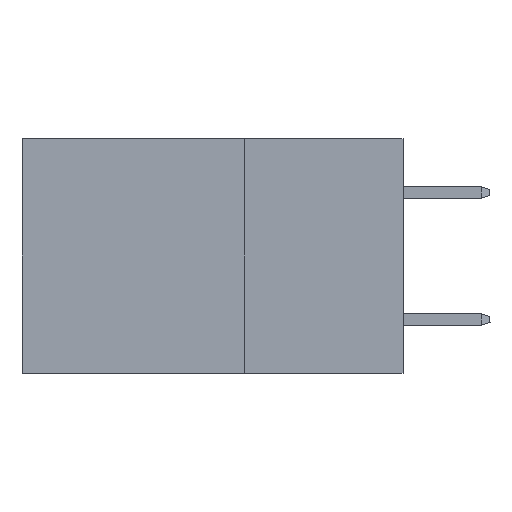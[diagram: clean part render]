
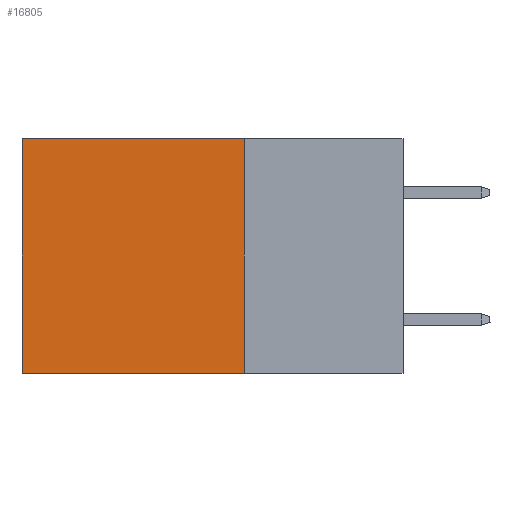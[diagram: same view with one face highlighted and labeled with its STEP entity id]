
A CAD part, left-side view. The second image highlights one B-rep face of the part: STEP entity #16805.
In plain terms, the highlighted planar face has unit normal (-1, 0, 0).
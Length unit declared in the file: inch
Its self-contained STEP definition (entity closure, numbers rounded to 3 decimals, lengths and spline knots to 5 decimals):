
#731 = CARTESIAN_POINT ( 'NONE',  ( 0.2875, 0.25, -0.37 ) ) ;
#1231 = EDGE_CURVE ( 'NONE', #6450, #15785, #3109, .T. ) ;
#1789 = VECTOR ( 'NONE', #8354, 39.37008 ) ;
#1845 = DIRECTION ( 'NONE',  ( 0., 0., -1. ) ) ;
#2257 = CARTESIAN_POINT ( 'NONE',  ( 0.2875, 0.25, -0.37 ) ) ;
#2353 = LINE ( 'NONE', #10045, #1789 ) ;
#3051 = AXIS2_PLACEMENT_3D ( 'NONE', #13558, #13741, #1845 ) ;
#3069 = CARTESIAN_POINT ( 'NONE',  ( 0.2875, 0.6, 0. ) ) ;
#3109 = LINE ( 'NONE', #10684, #17189 ) ;
#4097 = EDGE_CURVE ( 'NONE', #10694, #15785, #6699, .T. ) ;
#6450 = VERTEX_POINT ( 'NONE', #3069 ) ;
#6531 = ORIENTED_EDGE ( 'NONE', *, *, #14294, .F. ) ;
#6699 = LINE ( 'NONE', #2257, #8465 ) ;
#6700 = CARTESIAN_POINT ( 'NONE',  ( 0.2875, 0.25, 0. ) ) ;
#7744 = FACE_OUTER_BOUND ( 'NONE', #19006, .T. ) ;
#7772 = LINE ( 'NONE', #6700, #17917 ) ;
#7951 = ORIENTED_EDGE ( 'NONE', *, *, #18372, .T. ) ;
#8354 = DIRECTION ( 'NONE',  ( 0., 1., 0. ) ) ;
#8465 = VECTOR ( 'NONE', #18962, 39.37008 ) ;
#8827 = CARTESIAN_POINT ( 'NONE',  ( 0.2875, 0.6, -0.37 ) ) ;
#9132 = PLANE ( 'NONE',  #3051 ) ;
#10045 = CARTESIAN_POINT ( 'NONE',  ( 0.2875, 0.25, 0. ) ) ;
#10684 = CARTESIAN_POINT ( 'NONE',  ( 0.2875, 0.6, 0. ) ) ;
#10694 = VERTEX_POINT ( 'NONE', #731 ) ;
#12313 = DIRECTION ( 'NONE',  ( 0., 0., -1. ) ) ;
#13558 = CARTESIAN_POINT ( 'NONE',  ( 0.2875, 0.25, 0. ) ) ;
#13741 = DIRECTION ( 'NONE',  ( 1., 0., 0. ) ) ;
#14294 = EDGE_CURVE ( 'NONE', #16333, #10694, #7772, .T. ) ;
#14504 = ORIENTED_EDGE ( 'NONE', *, *, #4097, .F. ) ;
#15785 = VERTEX_POINT ( 'NONE', #8827 ) ;
#16333 = VERTEX_POINT ( 'NONE', #19385 ) ;
#16671 = DIRECTION ( 'NONE',  ( 0., 0., -1. ) ) ;
#16805 = ADVANCED_FACE ( 'NONE', ( #7744 ), #9132, .F. ) ;
#17189 = VECTOR ( 'NONE', #16671, 39.37008 ) ;
#17917 = VECTOR ( 'NONE', #12313, 39.37008 ) ;
#18372 = EDGE_CURVE ( 'NONE', #16333, #6450, #2353, .T. ) ;
#18438 = ORIENTED_EDGE ( 'NONE', *, *, #1231, .T. ) ;
#18962 = DIRECTION ( 'NONE',  ( 0., 1., 0. ) ) ;
#19006 = EDGE_LOOP ( 'NONE', ( #18438, #14504, #6531, #7951 ) ) ;
#19385 = CARTESIAN_POINT ( 'NONE',  ( 0.2875, 0.25, 0. ) ) ;
